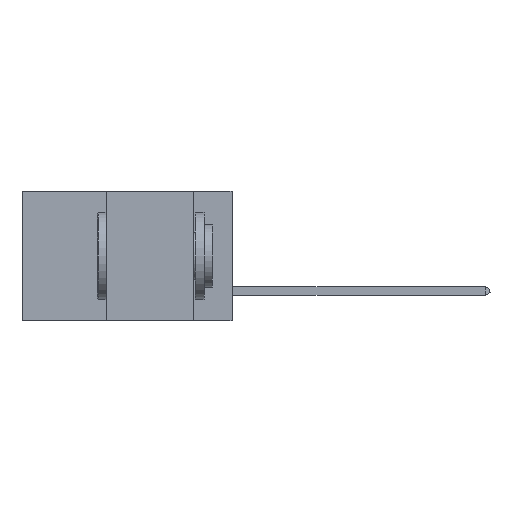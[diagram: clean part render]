
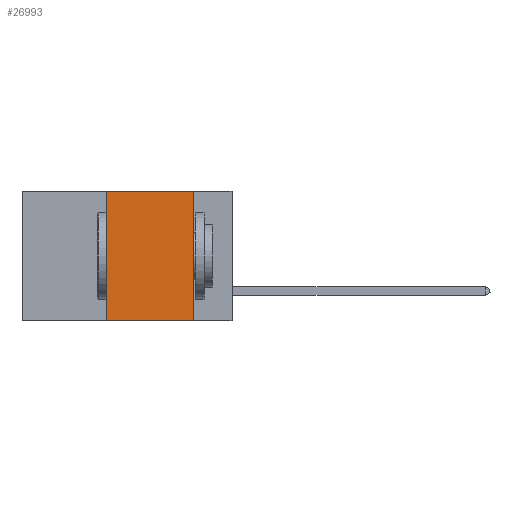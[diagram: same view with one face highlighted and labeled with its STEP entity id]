
A CAD part, left-side view. The second image highlights one B-rep face of the part: STEP entity #26993.
In plain terms, the highlighted planar face has unit normal (-1, 0, 0).
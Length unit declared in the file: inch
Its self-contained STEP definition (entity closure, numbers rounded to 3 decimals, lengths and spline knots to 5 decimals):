
#1043 = ORIENTED_EDGE ( 'NONE', *, *, #48361, .F. ) ;
#1139 = DIRECTION ( 'NONE',  ( 1., 0., 0. ) ) ;
#4340 = ORIENTED_EDGE ( 'NONE', *, *, #33982, .F. ) ;
#5015 = EDGE_CURVE ( 'NONE', #16402, #16031, #48520, .T. ) ;
#7935 = VERTEX_POINT ( 'NONE', #48417 ) ;
#12153 = EDGE_LOOP ( 'NONE', ( #4340, #1043, #23087, #18978 ) ) ;
#12918 = CARTESIAN_POINT ( 'NONE',  ( 0., 0.6, 0. ) ) ;
#16031 = VERTEX_POINT ( 'NONE', #38542 ) ;
#16402 = VERTEX_POINT ( 'NONE', #21463 ) ;
#16979 = DIRECTION ( 'NONE',  ( 0., -1., 0. ) ) ;
#18978 = ORIENTED_EDGE ( 'NONE', *, *, #5015, .T. ) ;
#19086 = CARTESIAN_POINT ( 'NONE',  ( 0., 0.11, 0. ) ) ;
#20181 = DIRECTION ( 'NONE',  ( 0., 0., -1. ) ) ;
#21463 = CARTESIAN_POINT ( 'NONE',  ( 0., 0.36, -0.37 ) ) ;
#23087 = ORIENTED_EDGE ( 'NONE', *, *, #40882, .F. ) ;
#25936 = LINE ( 'NONE', #45685, #37226 ) ;
#26993 = ADVANCED_FACE ( 'NONE', ( #35843 ), #31262, .F. ) ;
#27094 = VERTEX_POINT ( 'NONE', #40067 ) ;
#31262 = PLANE ( 'NONE',  #43666 ) ;
#32944 = VECTOR ( 'NONE', #42163, 39.37008 ) ;
#33982 = EDGE_CURVE ( 'NONE', #27094, #16031, #42396, .T. ) ;
#35843 = FACE_OUTER_BOUND ( 'NONE', #12153, .T. ) ;
#37226 = VECTOR ( 'NONE', #39032, 39.37008 ) ;
#38542 = CARTESIAN_POINT ( 'NONE',  ( 0., 0.11, -0.37 ) ) ;
#39032 = DIRECTION ( 'NONE',  ( 0., 0., 1. ) ) ;
#40067 = CARTESIAN_POINT ( 'NONE',  ( 0., 0.11, 0. ) ) ;
#40882 = EDGE_CURVE ( 'NONE', #16402, #7935, #25936, .T. ) ;
#41829 = VECTOR ( 'NONE', #45595, 39.37008 ) ;
#42163 = DIRECTION ( 'NONE',  ( 0., -1., 0. ) ) ;
#42396 = LINE ( 'NONE', #19086, #41829 ) ;
#43666 = AXIS2_PLACEMENT_3D ( 'NONE', #12918, #1139, #20181 ) ;
#43959 = CARTESIAN_POINT ( 'NONE',  ( 0., 0.6, -0.37 ) ) ;
#44972 = VECTOR ( 'NONE', #16979, 39.37008 ) ;
#45595 = DIRECTION ( 'NONE',  ( 0., 0., -1. ) ) ;
#45685 = CARTESIAN_POINT ( 'NONE',  ( 0., 0.36, 0. ) ) ;
#46606 = LINE ( 'NONE', #49118, #32944 ) ;
#48361 = EDGE_CURVE ( 'NONE', #7935, #27094, #46606, .T. ) ;
#48417 = CARTESIAN_POINT ( 'NONE',  ( 0., 0.36, 0. ) ) ;
#48520 = LINE ( 'NONE', #43959, #44972 ) ;
#49118 = CARTESIAN_POINT ( 'NONE',  ( 0., 0.6, 0. ) ) ;
